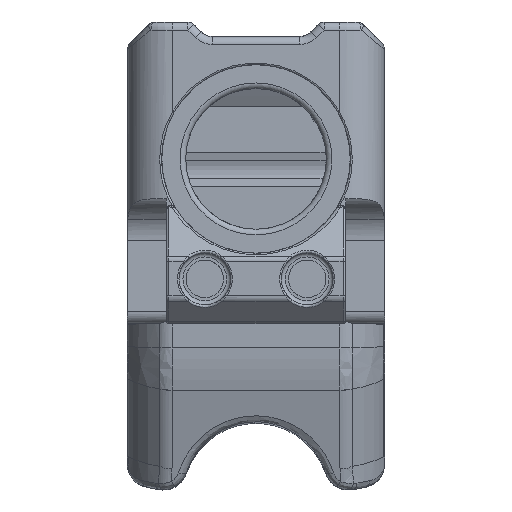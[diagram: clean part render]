
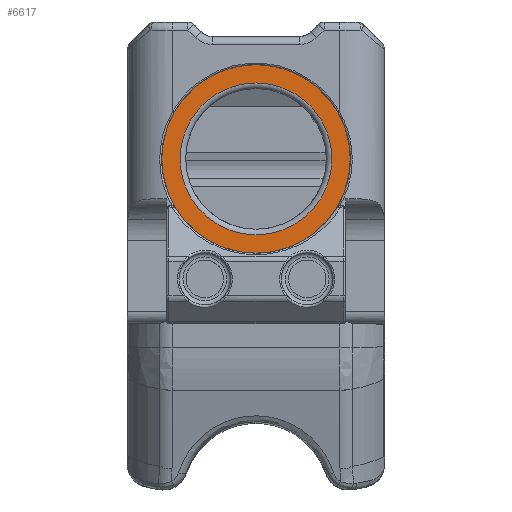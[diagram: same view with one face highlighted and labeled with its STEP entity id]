
A CAD part, front view. The second image highlights one B-rep face of the part: STEP entity #6617.
In plain terms, the highlighted planar face has unit normal (0, -1, 0).
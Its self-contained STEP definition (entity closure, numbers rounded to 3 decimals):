
#60=FACE_BOUND('',#1707,.T.);
#179=PLANE('',#7065);
#1288=FACE_OUTER_BOUND('',#1706,.T.);
#1706=EDGE_LOOP('',(#4548));
#1707=EDGE_LOOP('',(#4549));
#2126=CIRCLE('',#7064,9.425);
#2127=CIRCLE('',#7066,11.697);
#2763=VERTEX_POINT('',#10520);
#2764=VERTEX_POINT('',#10524);
#3440=EDGE_CURVE('',#2763,#2763,#2126,.T.);
#3441=EDGE_CURVE('',#2764,#2764,#2127,.T.);
#4548=ORIENTED_EDGE('',*,*,#3441,.T.);
#4549=ORIENTED_EDGE('',*,*,#3440,.F.);
#6617=ADVANCED_FACE('',(#1288,#60),#179,.T.);
#7064=AXIS2_PLACEMENT_3D('',#10522,#7917,#7918);
#7065=AXIS2_PLACEMENT_3D('',#10523,#7919,#7920);
#7066=AXIS2_PLACEMENT_3D('',#10525,#7921,#7922);
#7917=DIRECTION('center_axis',(0.,-1.,0.));
#7918=DIRECTION('ref_axis',(0.922,0.,0.388));
#7919=DIRECTION('center_axis',(0.,-1.,0.));
#7920=DIRECTION('ref_axis',(1.,0.,0.));
#7921=DIRECTION('center_axis',(0.,-1.,0.));
#7922=DIRECTION('ref_axis',(1.,0.,0.));
#10520=CARTESIAN_POINT('',(15.977,-18.733,-106.691));
#10522=CARTESIAN_POINT('Origin',(15.977,-18.733,-116.116));
#10523=CARTESIAN_POINT('Origin',(15.977,-18.733,-116.116));
#10524=CARTESIAN_POINT('',(15.977,-18.733,-127.813));
#10525=CARTESIAN_POINT('Origin',(15.977,-18.733,-116.116));
